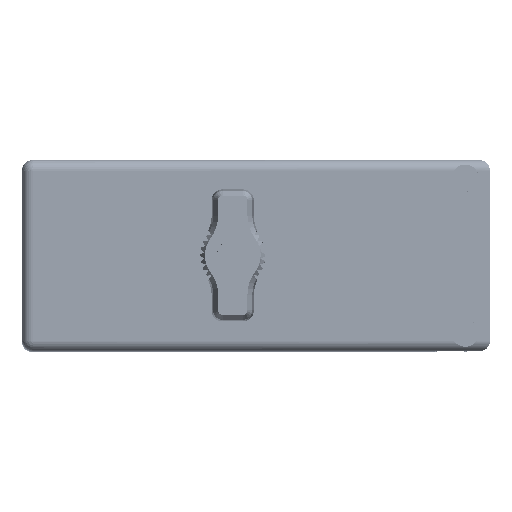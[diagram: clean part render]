
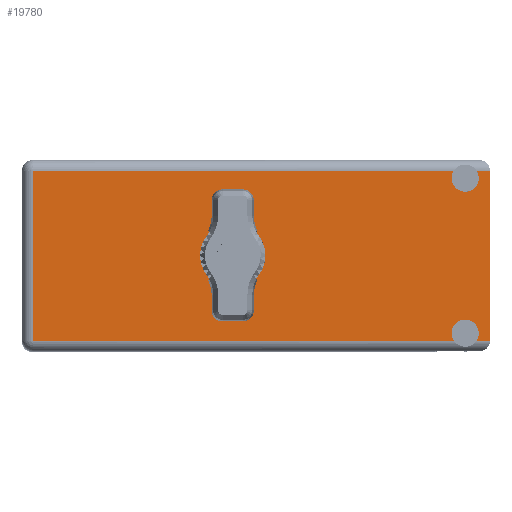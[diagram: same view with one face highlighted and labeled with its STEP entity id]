
A CAD part, top view. The second image highlights one B-rep face of the part: STEP entity #19780.
In plain terms, the highlighted face is planar.
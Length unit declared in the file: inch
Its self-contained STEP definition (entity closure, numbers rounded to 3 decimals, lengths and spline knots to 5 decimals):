
#248 = VERTEX_POINT ( 'NONE', #77451 ) ;
#670 = AXIS2_PLACEMENT_3D ( 'NONE', #26721, #19675, #47292 ) ;
#1356 = CIRCLE ( 'NONE', #22344, 0.125 ) ;
#1705 = CARTESIAN_POINT ( 'NONE',  ( 1.499, 1.675, 0.5 ) ) ;
#1884 = VERTEX_POINT ( 'NONE', #33295 ) ;
#2561 = DIRECTION ( 'NONE',  ( 0., 0., 1. ) ) ;
#5002 = VERTEX_POINT ( 'NONE', #26777 ) ;
#5104 = LINE ( 'NONE', #23996, #23858 ) ;
#5451 = CARTESIAN_POINT ( 'NONE',  ( 1.659, 1.675, 0.617 ) ) ;
#6163 = VECTOR ( 'NONE', #81307, 39.37008 ) ;
#6834 = AXIS2_PLACEMENT_3D ( 'NONE', #41355, #21181, #67214 ) ;
#8399 = CARTESIAN_POINT ( 'NONE',  ( 1.659, 1.675, 0.547 ) ) ;
#9989 = AXIS2_PLACEMENT_3D ( 'NONE', #61484, #50083, #29493 ) ;
#10427 = EDGE_CURVE ( 'NONE', #74990, #45645, #35693, .T. ) ;
#11817 = DIRECTION ( 'NONE',  ( 1., 0., 0. ) ) ;
#11893 = DIRECTION ( 'NONE',  ( -1., 0., 0. ) ) ;
#17203 = CARTESIAN_POINT ( 'NONE',  ( -1.289, 1.675, -0.547 ) ) ;
#17379 = ORIENTED_EDGE ( 'NONE', *, *, #24018, .T. ) ;
#18464 = CARTESIAN_POINT ( 'NONE',  ( -1.359, 1.675, -0.547 ) ) ;
#19675 = DIRECTION ( 'NONE',  ( 0., 1., 0. ) ) ;
#19780 = ADVANCED_FACE ( 'NONE', ( #34752, #36058 ), #82923, .T. ) ;
#21181 = DIRECTION ( 'NONE',  ( 0., 1., 0. ) ) ;
#21194 = EDGE_LOOP ( 'NONE', ( #64160, #59764, #82771, #71781, #71577, #17379, #58770, #28755, #30968, #35364 ) ) ;
#22344 = AXIS2_PLACEMENT_3D ( 'NONE', #33464, #80343, #26043 ) ;
#23858 = VECTOR ( 'NONE', #63444, 39.37008 ) ;
#23996 = CARTESIAN_POINT ( 'NONE',  ( -1.289, 1.675, -0.617 ) ) ;
#24018 = EDGE_CURVE ( 'NONE', #5002, #1884, #78492, .T. ) ;
#24216 = CARTESIAN_POINT ( 'NONE',  ( 1.659, 1.675, 0.547 ) ) ;
#24541 = CARTESIAN_POINT ( 'NONE',  ( 1.57281, 1.675, 0.547 ) ) ;
#24564 = LINE ( 'NONE', #45129, #65106 ) ;
#24915 = DIRECTION ( 'NONE',  ( 0., 1., 0. ) ) ;
#26043 = DIRECTION ( 'NONE',  ( 0., 0., 1. ) ) ;
#26721 = CARTESIAN_POINT ( 'NONE',  ( 1.499, 1.675, -0.5 ) ) ;
#26777 = CARTESIAN_POINT ( 'NONE',  ( 1.659, 1.675, -0.547 ) ) ;
#26919 = AXIS2_PLACEMENT_3D ( 'NONE', #58220, #24915, #84518 ) ;
#28755 = ORIENTED_EDGE ( 'NONE', *, *, #37177, .F. ) ;
#29493 = DIRECTION ( 'NONE',  ( -1., 0., 0. ) ) ;
#30968 = ORIENTED_EDGE ( 'NONE', *, *, #10427, .T. ) ;
#33295 = CARTESIAN_POINT ( 'NONE',  ( 1.57281, 1.675, -0.547 ) ) ;
#33464 = CARTESIAN_POINT ( 'NONE',  ( 0., 1.675, 0. ) ) ;
#34556 = VERTEX_POINT ( 'NONE', #24541 ) ;
#34752 = FACE_BOUND ( 'NONE', #85650, .T. ) ;
#35364 = ORIENTED_EDGE ( 'NONE', *, *, #68523, .T. ) ;
#35693 = LINE ( 'NONE', #69423, #42017 ) ;
#36058 = FACE_OUTER_BOUND ( 'NONE', #21194, .T. ) ;
#37177 = EDGE_CURVE ( 'NONE', #74990, #58714, #64668, .T. ) ;
#39289 = VERTEX_POINT ( 'NONE', #61954 ) ;
#39658 = LINE ( 'NONE', #5451, #57745 ) ;
#39763 = VERTEX_POINT ( 'NONE', #63893 ) ;
#40088 = DIRECTION ( 'NONE',  ( 0., 0., 1. ) ) ;
#41355 = CARTESIAN_POINT ( 'NONE',  ( 0., 1.675, 0. ) ) ;
#42017 = VECTOR ( 'NONE', #54553, 39.37008 ) ;
#43518 = EDGE_CURVE ( 'NONE', #39763, #44356, #52623, .T. ) ;
#44356 = VERTEX_POINT ( 'NONE', #74261 ) ;
#45129 = CARTESIAN_POINT ( 'NONE',  ( 1.659, 1.675, 0.547 ) ) ;
#45279 = VECTOR ( 'NONE', #11893, 39.37008 ) ;
#45645 = VERTEX_POINT ( 'NONE', #17203 ) ;
#45938 = ORIENTED_EDGE ( 'NONE', *, *, #79810, .F. ) ;
#47292 = DIRECTION ( 'NONE',  ( 0., 0., 1. ) ) ;
#47800 = DIRECTION ( 'NONE',  ( 0., 0., 1. ) ) ;
#48705 = ORIENTED_EDGE ( 'NONE', *, *, #67852, .F. ) ;
#50083 = DIRECTION ( 'NONE',  ( 0., 1., 0. ) ) ;
#52623 = CIRCLE ( 'NONE', #65240, 0.0875 ) ;
#54553 = DIRECTION ( 'NONE',  ( -1., 0., 0. ) ) ;
#55814 = CIRCLE ( 'NONE', #68439, 0.0875 ) ;
#57745 = VECTOR ( 'NONE', #40088, 39.37008 ) ;
#57893 = EDGE_CURVE ( 'NONE', #5002, #84105, #39658, .T. ) ;
#58220 = CARTESIAN_POINT ( 'NONE',  ( 1.499, 1.675, -0.5 ) ) ;
#58714 = VERTEX_POINT ( 'NONE', #64333 ) ;
#58770 = ORIENTED_EDGE ( 'NONE', *, *, #74701, .F. ) ;
#59764 = ORIENTED_EDGE ( 'NONE', *, *, #43518, .F. ) ;
#61484 = CARTESIAN_POINT ( 'NONE',  ( -1.359, 1.675, -0.617 ) ) ;
#61954 = CARTESIAN_POINT ( 'NONE',  ( -1.289, 1.675, 0.547 ) ) ;
#62248 = CIRCLE ( 'NONE', #670, 0.0875 ) ;
#62348 = EDGE_CURVE ( 'NONE', #39289, #44356, #24564, .T. ) ;
#63444 = DIRECTION ( 'NONE',  ( 0., 0., 1. ) ) ;
#63453 = CARTESIAN_POINT ( 'NONE',  ( 1.42519, 1.675, -0.547 ) ) ;
#63893 = CARTESIAN_POINT ( 'NONE',  ( 1.499, 1.675, 0.4125 ) ) ;
#64160 = ORIENTED_EDGE ( 'NONE', *, *, #62348, .T. ) ;
#64333 = CARTESIAN_POINT ( 'NONE',  ( 1.499, 1.675, -0.4125 ) ) ;
#64668 = CIRCLE ( 'NONE', #26919, 0.0875 ) ;
#65106 = VECTOR ( 'NONE', #11817, 39.37008 ) ;
#65240 = AXIS2_PLACEMENT_3D ( 'NONE', #1705, #83608, #2561 ) ;
#66469 = EDGE_CURVE ( 'NONE', #34556, #39763, #55814, .T. ) ;
#67214 = DIRECTION ( 'NONE',  ( 0., 0., 1. ) ) ;
#67852 = EDGE_CURVE ( 'NONE', #85051, #248, #1356, .T. ) ;
#68439 = AXIS2_PLACEMENT_3D ( 'NONE', #81506, #74072, #47800 ) ;
#68523 = EDGE_CURVE ( 'NONE', #45645, #39289, #5104, .T. ) ;
#69423 = CARTESIAN_POINT ( 'NONE',  ( -1.359, 1.675, -0.547 ) ) ;
#70663 = LINE ( 'NONE', #24216, #6163 ) ;
#71577 = ORIENTED_EDGE ( 'NONE', *, *, #57893, .F. ) ;
#71781 = ORIENTED_EDGE ( 'NONE', *, *, #75933, .T. ) ;
#73950 = CARTESIAN_POINT ( 'NONE',  ( 0., 1.675, -0.125 ) ) ;
#74072 = DIRECTION ( 'NONE',  ( 0., 1., 0. ) ) ;
#74261 = CARTESIAN_POINT ( 'NONE',  ( 1.42519, 1.675, 0.547 ) ) ;
#74701 = EDGE_CURVE ( 'NONE', #58714, #1884, #62248, .T. ) ;
#74990 = VERTEX_POINT ( 'NONE', #63453 ) ;
#75933 = EDGE_CURVE ( 'NONE', #34556, #84105, #70663, .T. ) ;
#77451 = CARTESIAN_POINT ( 'NONE',  ( 0., 1.675, 0.125 ) ) ;
#78492 = LINE ( 'NONE', #18464, #45279 ) ;
#79810 = EDGE_CURVE ( 'NONE', #248, #85051, #82603, .T. ) ;
#80343 = DIRECTION ( 'NONE',  ( 0., 1., 0. ) ) ;
#81307 = DIRECTION ( 'NONE',  ( 1., 0., 0. ) ) ;
#81506 = CARTESIAN_POINT ( 'NONE',  ( 1.499, 1.675, 0.5 ) ) ;
#82603 = CIRCLE ( 'NONE', #6834, 0.125 ) ;
#82771 = ORIENTED_EDGE ( 'NONE', *, *, #66469, .F. ) ;
#82923 = PLANE ( 'NONE',  #9989 ) ;
#83608 = DIRECTION ( 'NONE',  ( 0., 1., 0. ) ) ;
#84105 = VERTEX_POINT ( 'NONE', #8399 ) ;
#84518 = DIRECTION ( 'NONE',  ( 0., 0., 1. ) ) ;
#85051 = VERTEX_POINT ( 'NONE', #73950 ) ;
#85650 = EDGE_LOOP ( 'NONE', ( #45938, #48705 ) ) ;
